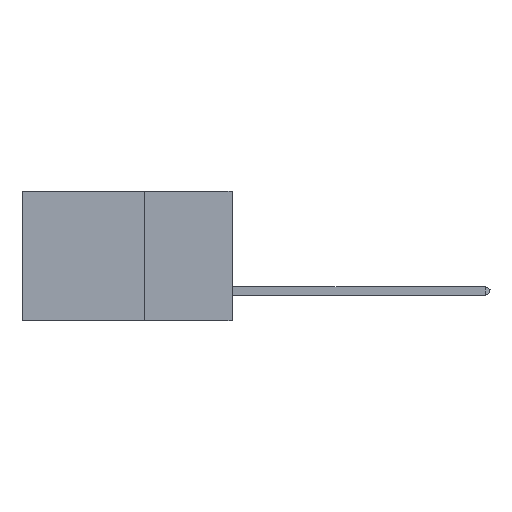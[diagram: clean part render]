
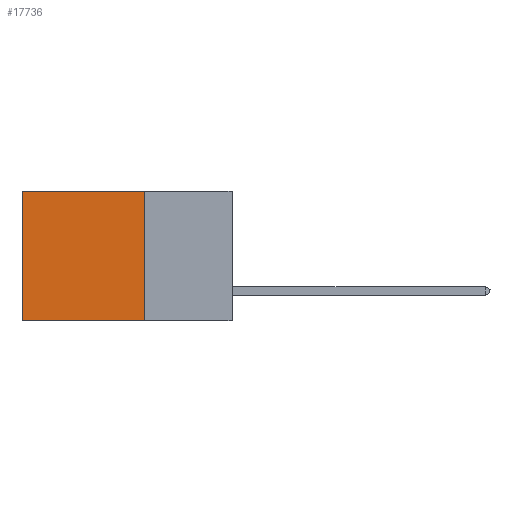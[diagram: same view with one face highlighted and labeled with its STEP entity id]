
A CAD part, left-side view. The second image highlights one B-rep face of the part: STEP entity #17736.
In plain terms, the highlighted planar face has unit normal (-1, 0, 0).
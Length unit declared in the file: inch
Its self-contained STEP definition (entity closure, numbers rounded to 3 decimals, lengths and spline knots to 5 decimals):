
#66 = DIRECTION ( 'NONE',  ( 0., 0., -1. ) ) ;
#899 = LINE ( 'NONE', #22653, #16345 ) ;
#2812 = CARTESIAN_POINT ( 'NONE',  ( 0.2875, 0.25, -0.37 ) ) ;
#3042 = CARTESIAN_POINT ( 'NONE',  ( 0.2875, 0.25, 0. ) ) ;
#3429 = LINE ( 'NONE', #4275, #19191 ) ;
#3843 = PLANE ( 'NONE',  #6624 ) ;
#4275 = CARTESIAN_POINT ( 'NONE',  ( 0.2875, 0.6, 0. ) ) ;
#5531 = VERTEX_POINT ( 'NONE', #18613 ) ;
#6050 = VERTEX_POINT ( 'NONE', #2812 ) ;
#6397 = CARTESIAN_POINT ( 'NONE',  ( 0.2875, 0.25, 0. ) ) ;
#6624 = AXIS2_PLACEMENT_3D ( 'NONE', #6397, #15622, #6829 ) ;
#6829 = DIRECTION ( 'NONE',  ( 0., 0., -1. ) ) ;
#7351 = VERTEX_POINT ( 'NONE', #21783 ) ;
#8916 = FACE_OUTER_BOUND ( 'NONE', #18231, .T. ) ;
#10451 = EDGE_CURVE ( 'NONE', #6050, #7351, #10771, .T. ) ;
#10648 = ORIENTED_EDGE ( 'NONE', *, *, #21182, .F. ) ;
#10771 = LINE ( 'NONE', #14936, #15166 ) ;
#11503 = ORIENTED_EDGE ( 'NONE', *, *, #16034, .T. ) ;
#14936 = CARTESIAN_POINT ( 'NONE',  ( 0.2875, 0.25, -0.37 ) ) ;
#15166 = VECTOR ( 'NONE', #16765, 39.37008 ) ;
#15622 = DIRECTION ( 'NONE',  ( 1., 0., 0. ) ) ;
#15796 = ORIENTED_EDGE ( 'NONE', *, *, #10451, .F. ) ;
#15856 = ORIENTED_EDGE ( 'NONE', *, *, #24285, .T. ) ;
#16034 = EDGE_CURVE ( 'NONE', #18542, #5531, #21177, .T. ) ;
#16345 = VECTOR ( 'NONE', #66, 39.37008 ) ;
#16765 = DIRECTION ( 'NONE',  ( 0., 1., 0. ) ) ;
#17736 = ADVANCED_FACE ( 'NONE', ( #8916 ), #3843, .F. ) ;
#17945 = CARTESIAN_POINT ( 'NONE',  ( 0.2875, 0.25, 0. ) ) ;
#18231 = EDGE_LOOP ( 'NONE', ( #15856, #15796, #10648, #11503 ) ) ;
#18542 = VERTEX_POINT ( 'NONE', #17945 ) ;
#18613 = CARTESIAN_POINT ( 'NONE',  ( 0.2875, 0.6, 0. ) ) ;
#19191 = VECTOR ( 'NONE', #23477, 39.37008 ) ;
#21177 = LINE ( 'NONE', #3042, #23573 ) ;
#21182 = EDGE_CURVE ( 'NONE', #18542, #6050, #899, .T. ) ;
#21716 = DIRECTION ( 'NONE',  ( 0., 1., 0. ) ) ;
#21783 = CARTESIAN_POINT ( 'NONE',  ( 0.2875, 0.6, -0.37 ) ) ;
#22653 = CARTESIAN_POINT ( 'NONE',  ( 0.2875, 0.25, 0. ) ) ;
#23477 = DIRECTION ( 'NONE',  ( 0., 0., -1. ) ) ;
#23573 = VECTOR ( 'NONE', #21716, 39.37008 ) ;
#24285 = EDGE_CURVE ( 'NONE', #5531, #7351, #3429, .T. ) ;
